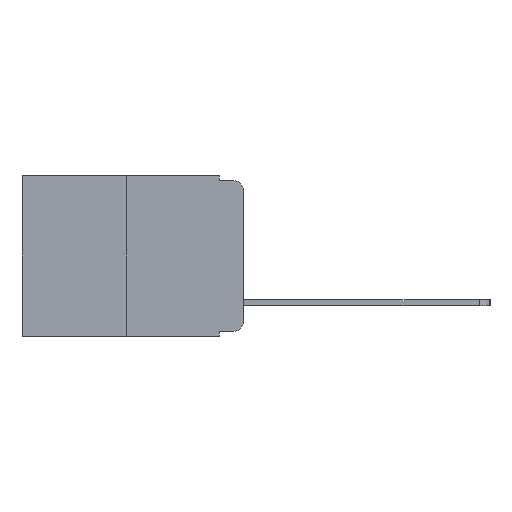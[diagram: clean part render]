
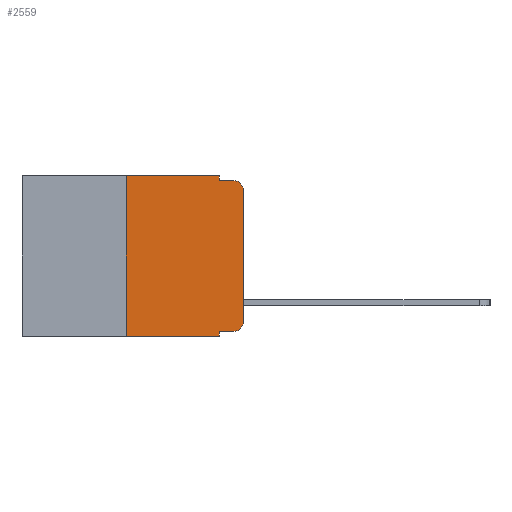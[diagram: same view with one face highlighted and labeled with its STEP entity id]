
A CAD part, left-side view. The second image highlights one B-rep face of the part: STEP entity #2559.
In plain terms, the highlighted planar face has unit normal (-1, 0, 0).
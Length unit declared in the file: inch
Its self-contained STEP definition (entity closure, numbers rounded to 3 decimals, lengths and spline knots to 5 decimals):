
#867 = VERTEX_POINT ( 'NONE', #13639 ) ;
#994 = VECTOR ( 'NONE', #9526, 39.37008 ) ;
#1243 = VERTEX_POINT ( 'NONE', #6032 ) ;
#1505 = CARTESIAN_POINT ( 'NONE',  ( 0., 0.25, 0. ) ) ;
#1948 = ORIENTED_EDGE ( 'NONE', *, *, #18086, .T. ) ;
#1968 = DIRECTION ( 'NONE',  ( 0., -1., 0. ) ) ;
#2407 = ORIENTED_EDGE ( 'NONE', *, *, #13779, .F. ) ;
#2559 = ADVANCED_FACE ( 'NONE', ( #9591 ), #12521, .F. ) ;
#2878 = ORIENTED_EDGE ( 'NONE', *, *, #4452, .F. ) ;
#3046 = CARTESIAN_POINT ( 'NONE',  ( 0., 0.473, 0. ) ) ;
#3879 = ORIENTED_EDGE ( 'NONE', *, *, #14817, .F. ) ;
#4014 = CARTESIAN_POINT ( 'NONE',  ( 0., 0.051, -0.01 ) ) ;
#4037 = LINE ( 'NONE', #4014, #16030 ) ;
#4452 = EDGE_CURVE ( 'NONE', #15852, #18214, #15497, .T. ) ;
#4544 = DIRECTION ( 'NONE',  ( 0., 0., -1. ) ) ;
#4632 = VECTOR ( 'NONE', #1968, 39.37008 ) ;
#4659 = DIRECTION ( 'NONE',  ( 1., 0., 0. ) ) ;
#4937 = VECTOR ( 'NONE', #4544, 39.37008 ) ;
#5100 = ORIENTED_EDGE ( 'NONE', *, *, #15830, .F. ) ;
#5133 = CARTESIAN_POINT ( 'NONE',  ( 0., 0.051, -0.333 ) ) ;
#5174 = CARTESIAN_POINT ( 'NONE',  ( 0., 0.051, -0.333 ) ) ;
#5436 = CARTESIAN_POINT ( 'NONE',  ( 0., 0.02, -0.333 ) ) ;
#5473 = CARTESIAN_POINT ( 'NONE',  ( 0., 0.051, -0.343 ) ) ;
#5627 = DIRECTION ( 'NONE',  ( 0., -1., 0. ) ) ;
#5872 = ORIENTED_EDGE ( 'NONE', *, *, #16821, .T. ) ;
#5999 = ORIENTED_EDGE ( 'NONE', *, *, #17825, .T. ) ;
#6032 = CARTESIAN_POINT ( 'NONE',  ( 0., 0.051, -0.01 ) ) ;
#6052 = AXIS2_PLACEMENT_3D ( 'NONE', #3046, #4659, #15592 ) ;
#6234 = LINE ( 'NONE', #12361, #18062 ) ;
#6425 = CARTESIAN_POINT ( 'NONE',  ( 0., 0., -0.313 ) ) ;
#6716 = CARTESIAN_POINT ( 'NONE',  ( 0., 0.02, -0.03 ) ) ;
#7482 = CARTESIAN_POINT ( 'NONE',  ( 0., 0.02, -0.313 ) ) ;
#7740 = ORIENTED_EDGE ( 'NONE', *, *, #11758, .T. ) ;
#7813 = CARTESIAN_POINT ( 'NONE',  ( 0., 0.051, 0. ) ) ;
#8319 = ORIENTED_EDGE ( 'NONE', *, *, #10722, .T. ) ;
#8371 = DIRECTION ( 'NONE',  ( 0., 0., -1. ) ) ;
#8558 = ORIENTED_EDGE ( 'NONE', *, *, #12765, .F. ) ;
#8638 = EDGE_LOOP ( 'NONE', ( #5999, #5872, #5100, #3879, #2878, #2407, #1948, #8558, #7740, #8319 ) ) ;
#8653 = VERTEX_POINT ( 'NONE', #18792 ) ;
#9077 = CARTESIAN_POINT ( 'NONE',  ( 0., 0.051, 0. ) ) ;
#9108 = DIRECTION ( 'NONE',  ( 0., 0., -1. ) ) ;
#9526 = DIRECTION ( 'NONE',  ( 0., 0., 1. ) ) ;
#9591 = FACE_OUTER_BOUND ( 'NONE', #8638, .T. ) ;
#9732 = LINE ( 'NONE', #7813, #4937 ) ;
#9768 = VECTOR ( 'NONE', #11831, 39.37008 ) ;
#9780 = VERTEX_POINT ( 'NONE', #17236 ) ;
#9825 = CIRCLE ( 'NONE', #14857, 0.02 ) ;
#10007 = LINE ( 'NONE', #1505, #994 ) ;
#10293 = CARTESIAN_POINT ( 'NONE',  ( 0., 0.473, -0.343 ) ) ;
#10445 = CARTESIAN_POINT ( 'NONE',  ( 0., 0.25, 0. ) ) ;
#10722 = EDGE_CURVE ( 'NONE', #20044, #16720, #19144, .T. ) ;
#10783 = DIRECTION ( 'NONE',  ( 0., 0., -1. ) ) ;
#11078 = VERTEX_POINT ( 'NONE', #5133 ) ;
#11202 = VERTEX_POINT ( 'NONE', #5473 ) ;
#11758 = EDGE_CURVE ( 'NONE', #11078, #20044, #13019, .T. ) ;
#11831 = DIRECTION ( 'NONE',  ( 0., -1., 0. ) ) ;
#12327 = AXIS2_PLACEMENT_3D ( 'NONE', #7482, #18193, #9108 ) ;
#12361 = CARTESIAN_POINT ( 'NONE',  ( 0., 0., 0. ) ) ;
#12521 = PLANE ( 'NONE',  #6052 ) ;
#12729 = CARTESIAN_POINT ( 'NONE',  ( 0., 0.473, 0. ) ) ;
#12765 = EDGE_CURVE ( 'NONE', #11078, #11202, #13399, .T. ) ;
#13019 = LINE ( 'NONE', #5174, #4632 ) ;
#13399 = LINE ( 'NONE', #13845, #19513 ) ;
#13639 = CARTESIAN_POINT ( 'NONE',  ( 0., 0., -0.03 ) ) ;
#13779 = EDGE_CURVE ( 'NONE', #9780, #15852, #10007, .T. ) ;
#13803 = LINE ( 'NONE', #10293, #9768 ) ;
#13845 = CARTESIAN_POINT ( 'NONE',  ( 0., 0.051, 0. ) ) ;
#14260 = DIRECTION ( 'NONE',  ( 0., -1., 0. ) ) ;
#14817 = EDGE_CURVE ( 'NONE', #18214, #1243, #9732, .T. ) ;
#14857 = AXIS2_PLACEMENT_3D ( 'NONE', #6716, #17479, #8371 ) ;
#15426 = DIRECTION ( 'NONE',  ( 0., 0., 1. ) ) ;
#15497 = LINE ( 'NONE', #12729, #18995 ) ;
#15592 = DIRECTION ( 'NONE',  ( 0., 0., -1. ) ) ;
#15830 = EDGE_CURVE ( 'NONE', #1243, #8653, #4037, .T. ) ;
#15852 = VERTEX_POINT ( 'NONE', #10445 ) ;
#16030 = VECTOR ( 'NONE', #5627, 39.37008 ) ;
#16720 = VERTEX_POINT ( 'NONE', #6425 ) ;
#16821 = EDGE_CURVE ( 'NONE', #867, #8653, #9825, .T. ) ;
#17236 = CARTESIAN_POINT ( 'NONE',  ( 0., 0.25, -0.343 ) ) ;
#17479 = DIRECTION ( 'NONE',  ( -1., 0., 0. ) ) ;
#17825 = EDGE_CURVE ( 'NONE', #16720, #867, #6234, .T. ) ;
#18062 = VECTOR ( 'NONE', #15426, 39.37008 ) ;
#18086 = EDGE_CURVE ( 'NONE', #9780, #11202, #13803, .T. ) ;
#18193 = DIRECTION ( 'NONE',  ( -1., 0., 0. ) ) ;
#18214 = VERTEX_POINT ( 'NONE', #9077 ) ;
#18792 = CARTESIAN_POINT ( 'NONE',  ( 0., 0.02, -0.01 ) ) ;
#18995 = VECTOR ( 'NONE', #14260, 39.37008 ) ;
#19144 = CIRCLE ( 'NONE', #12327, 0.02 ) ;
#19513 = VECTOR ( 'NONE', #10783, 39.37008 ) ;
#20044 = VERTEX_POINT ( 'NONE', #5436 ) ;
